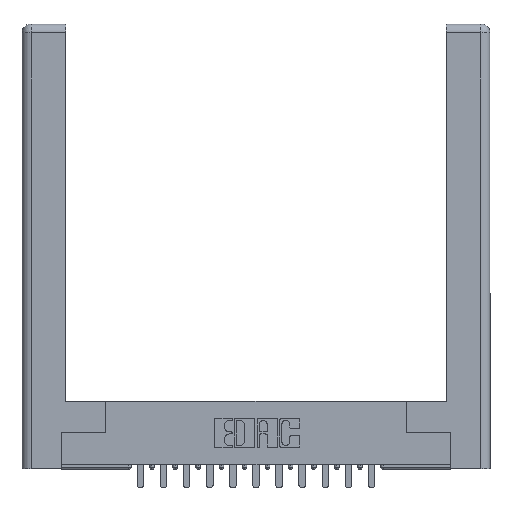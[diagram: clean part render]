
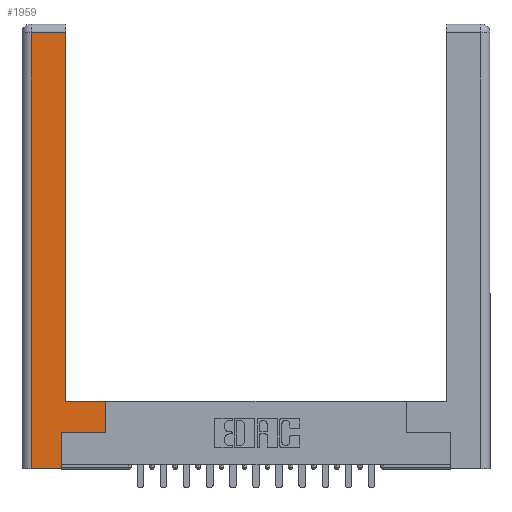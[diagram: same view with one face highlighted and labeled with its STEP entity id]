
A CAD part, top view. The second image highlights one B-rep face of the part: STEP entity #1959.
In plain terms, the highlighted planar face has unit normal (0, 0, 1).
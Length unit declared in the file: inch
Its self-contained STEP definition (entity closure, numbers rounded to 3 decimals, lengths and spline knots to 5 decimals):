
#386 = ORIENTED_EDGE ( 'NONE', *, *, #4089, .T. ) ;
#674 = DIRECTION ( 'NONE',  ( 1., 0., 0. ) ) ;
#1391 = ORIENTED_EDGE ( 'NONE', *, *, #4880, .T. ) ;
#1495 = CARTESIAN_POINT ( 'NONE',  ( 0.265, 0., 0. ) ) ;
#1521 = ORIENTED_EDGE ( 'NONE', *, *, #13405, .T. ) ;
#1959 = ADVANCED_FACE ( 'NONE', ( #8017 ), #10285, .F. ) ;
#1977 = CARTESIAN_POINT ( 'NONE',  ( 0.565, 0.245, 0. ) ) ;
#2176 = VERTEX_POINT ( 'NONE', #17250 ) ;
#2904 = CARTESIAN_POINT ( 'NONE',  ( 0.565, 0.45, 0. ) ) ;
#3217 = DIRECTION ( 'NONE',  ( 0., 1., 0. ) ) ;
#3277 = ORIENTED_EDGE ( 'NONE', *, *, #5139, .T. ) ;
#4089 = EDGE_CURVE ( 'NONE', #17926, #14099, #8258, .T. ) ;
#4375 = LINE ( 'NONE', #12024, #8270 ) ;
#4381 = CARTESIAN_POINT ( 'NONE',  ( 0.295, 0.45, 0. ) ) ;
#4437 = DIRECTION ( 'NONE',  ( 0., 1., 0. ) ) ;
#4465 = CARTESIAN_POINT ( 'NONE',  ( 0.265, 0.245, 0. ) ) ;
#4597 = CARTESIAN_POINT ( 'NONE',  ( 0.0615, 2.94, 0. ) ) ;
#4733 = LINE ( 'NONE', #9043, #7988 ) ;
#4880 = EDGE_CURVE ( 'NONE', #5062, #18104, #4733, .T. ) ;
#4947 = ORIENTED_EDGE ( 'NONE', *, *, #9739, .T. ) ;
#5062 = VERTEX_POINT ( 'NONE', #17665 ) ;
#5090 = DIRECTION ( 'NONE',  ( 0., 0., -1. ) ) ;
#5108 = LINE ( 'NONE', #2904, #8174 ) ;
#5139 = EDGE_CURVE ( 'NONE', #14099, #17504, #17036, .T. ) ;
#5250 = DIRECTION ( 'NONE',  ( 1., 0., 0. ) ) ;
#5511 = CARTESIAN_POINT ( 'NONE',  ( 0.295, 3., 0. ) ) ;
#5582 = VERTEX_POINT ( 'NONE', #14413 ) ;
#5716 = VECTOR ( 'NONE', #8373, 39.37008 ) ;
#5725 = DIRECTION ( 'NONE',  ( -1., 0., 0. ) ) ;
#5849 = EDGE_LOOP ( 'NONE', ( #12129, #1521, #386, #3277, #7397, #1391, #4947, #11899 ) ) ;
#7019 = LINE ( 'NONE', #4381, #17617 ) ;
#7157 = VECTOR ( 'NONE', #16714, 39.37008 ) ;
#7397 = ORIENTED_EDGE ( 'NONE', *, *, #7634, .T. ) ;
#7634 = EDGE_CURVE ( 'NONE', #17504, #5062, #8330, .T. ) ;
#7988 = VECTOR ( 'NONE', #674, 39.37008 ) ;
#8017 = FACE_OUTER_BOUND ( 'NONE', #5849, .T. ) ;
#8174 = VECTOR ( 'NONE', #4437, 39.37008 ) ;
#8258 = LINE ( 'NONE', #15244, #7157 ) ;
#8270 = VECTOR ( 'NONE', #13369, 39.37008 ) ;
#8330 = LINE ( 'NONE', #4465, #16484 ) ;
#8373 = DIRECTION ( 'NONE',  ( 0., 1., 0. ) ) ;
#9043 = CARTESIAN_POINT ( 'NONE',  ( 0.565, 0.245, 0. ) ) ;
#9739 = EDGE_CURVE ( 'NONE', #18104, #14401, #5108, .T. ) ;
#10285 = PLANE ( 'NONE',  #11664 ) ;
#11092 = EDGE_CURVE ( 'NONE', #14401, #5582, #7019, .T. ) ;
#11664 = AXIS2_PLACEMENT_3D ( 'NONE', #11714, #5090, #16205 ) ;
#11714 = CARTESIAN_POINT ( 'NONE',  ( 0., 0., 0. ) ) ;
#11794 = CARTESIAN_POINT ( 'NONE',  ( 0.265, 0., 0. ) ) ;
#11899 = ORIENTED_EDGE ( 'NONE', *, *, #11092, .T. ) ;
#12024 = CARTESIAN_POINT ( 'NONE',  ( 0.0615, 2.94, 0. ) ) ;
#12102 = CARTESIAN_POINT ( 'NONE',  ( 0.0615, 0., 0. ) ) ;
#12129 = ORIENTED_EDGE ( 'NONE', *, *, #12356, .T. ) ;
#12356 = EDGE_CURVE ( 'NONE', #5582, #2176, #14743, .T. ) ;
#13335 = VECTOR ( 'NONE', #5250, 39.37008 ) ;
#13369 = DIRECTION ( 'NONE',  ( -1., 0., 0. ) ) ;
#13405 = EDGE_CURVE ( 'NONE', #2176, #17926, #4375, .T. ) ;
#14099 = VERTEX_POINT ( 'NONE', #12102 ) ;
#14401 = VERTEX_POINT ( 'NONE', #18194 ) ;
#14413 = CARTESIAN_POINT ( 'NONE',  ( 0.295, 0.45, 0. ) ) ;
#14743 = LINE ( 'NONE', #5511, #5716 ) ;
#15244 = CARTESIAN_POINT ( 'NONE',  ( 0.0615, 0., 0. ) ) ;
#16205 = DIRECTION ( 'NONE',  ( -1., 0., 0. ) ) ;
#16484 = VECTOR ( 'NONE', #3217, 39.37008 ) ;
#16714 = DIRECTION ( 'NONE',  ( 0., -1., 0. ) ) ;
#17036 = LINE ( 'NONE', #1495, #13335 ) ;
#17250 = CARTESIAN_POINT ( 'NONE',  ( 0.295, 2.94, 0. ) ) ;
#17504 = VERTEX_POINT ( 'NONE', #11794 ) ;
#17617 = VECTOR ( 'NONE', #5725, 39.37008 ) ;
#17665 = CARTESIAN_POINT ( 'NONE',  ( 0.265, 0.245, 0. ) ) ;
#17926 = VERTEX_POINT ( 'NONE', #4597 ) ;
#18104 = VERTEX_POINT ( 'NONE', #1977 ) ;
#18194 = CARTESIAN_POINT ( 'NONE',  ( 0.565, 0.45, 0. ) ) ;
